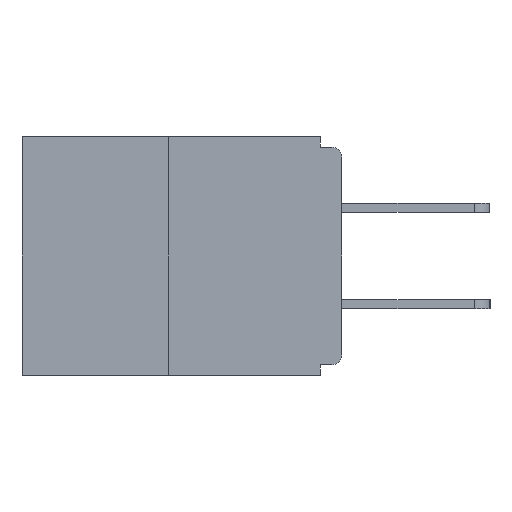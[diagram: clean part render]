
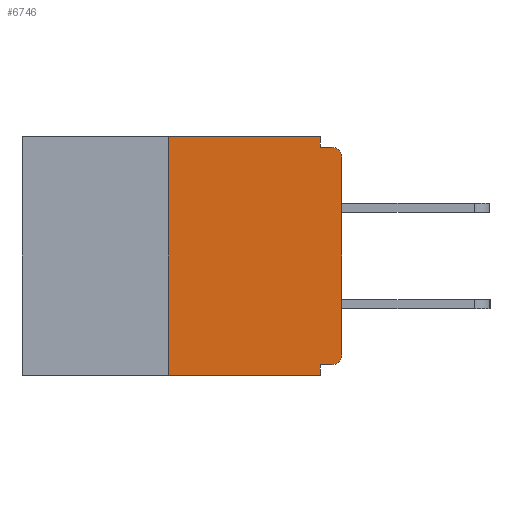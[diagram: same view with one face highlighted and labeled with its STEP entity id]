
A CAD part, left-side view. The second image highlights one B-rep face of the part: STEP entity #6746.
In plain terms, the highlighted planar face has unit normal (-1, 0, 0).
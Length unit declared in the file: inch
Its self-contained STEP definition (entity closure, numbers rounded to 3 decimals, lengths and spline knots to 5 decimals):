
#115 = EDGE_LOOP ( 'NONE', ( #3226, #12368, #12212, #9473, #7868, #4380, #4260, #8943, #7143, #5866 ) ) ;
#445 = DIRECTION ( 'NONE',  ( 0., -1., 0. ) ) ;
#654 = VECTOR ( 'NONE', #9874, 39.37008 ) ;
#875 = CARTESIAN_POINT ( 'NONE',  ( 0., 0., 0. ) ) ;
#1223 = EDGE_CURVE ( 'NONE', #3018, #7444, #6487, .T. ) ;
#1386 = VERTEX_POINT ( 'NONE', #5911 ) ;
#1626 = CARTESIAN_POINT ( 'NONE',  ( 0., 0., -0.03 ) ) ;
#1693 = CIRCLE ( 'NONE', #7611, 0.015 ) ;
#1786 = VECTOR ( 'NONE', #445, 39.37008 ) ;
#2025 = VERTEX_POINT ( 'NONE', #10905 ) ;
#2146 = CARTESIAN_POINT ( 'NONE',  ( 0., 0.015, -0.015 ) ) ;
#2231 = EDGE_CURVE ( 'NONE', #6453, #13157, #6046, .T. ) ;
#2232 = EDGE_CURVE ( 'NONE', #4487, #3018, #13692, .T. ) ;
#2355 = CARTESIAN_POINT ( 'NONE',  ( 0., 0.015, -0.03 ) ) ;
#2812 = DIRECTION ( 'NONE',  ( 0., 0., -1. ) ) ;
#2990 = LINE ( 'NONE', #7348, #11748 ) ;
#2993 = EDGE_CURVE ( 'NONE', #1386, #13157, #13668, .T. ) ;
#3010 = LINE ( 'NONE', #7367, #12233 ) ;
#3018 = VERTEX_POINT ( 'NONE', #1626 ) ;
#3226 = ORIENTED_EDGE ( 'NONE', *, *, #5640, .F. ) ;
#3436 = EDGE_CURVE ( 'NONE', #2025, #4487, #1693, .T. ) ;
#3664 = PLANE ( 'NONE',  #12753 ) ;
#3708 = EDGE_CURVE ( 'NONE', #8237, #4792, #5709, .T. ) ;
#3715 = VECTOR ( 'NONE', #2812, 39.37008 ) ;
#3766 = LINE ( 'NONE', #12398, #1786 ) ;
#3793 = DIRECTION ( 'NONE',  ( 1., 0., 0. ) ) ;
#4013 = EDGE_CURVE ( 'NONE', #4792, #7444, #9715, .T. ) ;
#4260 = ORIENTED_EDGE ( 'NONE', *, *, #2232, .T. ) ;
#4293 = DIRECTION ( 'NONE',  ( 0., 0., -1. ) ) ;
#4380 = ORIENTED_EDGE ( 'NONE', *, *, #3436, .T. ) ;
#4487 = VERTEX_POINT ( 'NONE', #13026 ) ;
#4792 = VERTEX_POINT ( 'NONE', #13716 ) ;
#4859 = CARTESIAN_POINT ( 'NONE',  ( 0., 0.46, 0. ) ) ;
#4881 = AXIS2_PLACEMENT_3D ( 'NONE', #2355, #11877, #13211 ) ;
#4924 = EDGE_CURVE ( 'NONE', #2025, #1386, #3010, .T. ) ;
#5147 = DIRECTION ( 'NONE',  ( -1., 0., 0. ) ) ;
#5640 = EDGE_CURVE ( 'NONE', #11037, #8237, #3766, .T. ) ;
#5709 = LINE ( 'NONE', #8798, #654 ) ;
#5866 = ORIENTED_EDGE ( 'NONE', *, *, #3708, .F. ) ;
#5911 = CARTESIAN_POINT ( 'NONE',  ( 0., 0.031, -0.328 ) ) ;
#6046 = LINE ( 'NONE', #7124, #10108 ) ;
#6074 = CARTESIAN_POINT ( 'NONE',  ( 0., 0.015, -0.313 ) ) ;
#6453 = VERTEX_POINT ( 'NONE', #7529 ) ;
#6487 = CIRCLE ( 'NONE', #4881, 0.015 ) ;
#6696 = CARTESIAN_POINT ( 'NONE',  ( 0., 0.25, 0. ) ) ;
#6746 = ADVANCED_FACE ( 'NONE', ( #9229 ), #3664, .F. ) ;
#7124 = CARTESIAN_POINT ( 'NONE',  ( 0., 0.46, -0.343 ) ) ;
#7143 = ORIENTED_EDGE ( 'NONE', *, *, #4013, .F. ) ;
#7348 = CARTESIAN_POINT ( 'NONE',  ( 0., 0.25, 0. ) ) ;
#7367 = CARTESIAN_POINT ( 'NONE',  ( 0., 0., -0.328 ) ) ;
#7444 = VERTEX_POINT ( 'NONE', #2146 ) ;
#7529 = CARTESIAN_POINT ( 'NONE',  ( 0., 0.25, -0.343 ) ) ;
#7544 = CARTESIAN_POINT ( 'NONE',  ( 0., 0.031, -0.343 ) ) ;
#7611 = AXIS2_PLACEMENT_3D ( 'NONE', #6074, #5147, #4293 ) ;
#7868 = ORIENTED_EDGE ( 'NONE', *, *, #4924, .F. ) ;
#8237 = VERTEX_POINT ( 'NONE', #9869 ) ;
#8421 = DIRECTION ( 'NONE',  ( 0., -1., 0. ) ) ;
#8643 = CARTESIAN_POINT ( 'NONE',  ( 0., 0., -0.015 ) ) ;
#8655 = DIRECTION ( 'NONE',  ( 0., 1., 0. ) ) ;
#8798 = CARTESIAN_POINT ( 'NONE',  ( 0., 0.031, 0. ) ) ;
#8943 = ORIENTED_EDGE ( 'NONE', *, *, #1223, .T. ) ;
#9164 = DIRECTION ( 'NONE',  ( 0., 0., -1. ) ) ;
#9229 = FACE_OUTER_BOUND ( 'NONE', #115, .T. ) ;
#9473 = ORIENTED_EDGE ( 'NONE', *, *, #2993, .F. ) ;
#9715 = LINE ( 'NONE', #8643, #11116 ) ;
#9869 = CARTESIAN_POINT ( 'NONE',  ( 0., 0.031, 0. ) ) ;
#9874 = DIRECTION ( 'NONE',  ( 0., 0., -1. ) ) ;
#10108 = VECTOR ( 'NONE', #8421, 39.37008 ) ;
#10905 = CARTESIAN_POINT ( 'NONE',  ( 0., 0.015, -0.328 ) ) ;
#10976 = EDGE_CURVE ( 'NONE', #6453, #11037, #2990, .T. ) ;
#11037 = VERTEX_POINT ( 'NONE', #6696 ) ;
#11116 = VECTOR ( 'NONE', #14056, 39.37008 ) ;
#11706 = DIRECTION ( 'NONE',  ( 0., 0., 1. ) ) ;
#11748 = VECTOR ( 'NONE', #11706, 39.37008 ) ;
#11877 = DIRECTION ( 'NONE',  ( -1., 0., 0. ) ) ;
#12212 = ORIENTED_EDGE ( 'NONE', *, *, #2231, .T. ) ;
#12233 = VECTOR ( 'NONE', #8655, 39.37008 ) ;
#12368 = ORIENTED_EDGE ( 'NONE', *, *, #10976, .F. ) ;
#12398 = CARTESIAN_POINT ( 'NONE',  ( 0., 0.46, 0. ) ) ;
#12753 = AXIS2_PLACEMENT_3D ( 'NONE', #4859, #3793, #9164 ) ;
#12764 = DIRECTION ( 'NONE',  ( 0., 0., 1. ) ) ;
#13026 = CARTESIAN_POINT ( 'NONE',  ( 0., 0., -0.313 ) ) ;
#13157 = VERTEX_POINT ( 'NONE', #7544 ) ;
#13211 = DIRECTION ( 'NONE',  ( 0., 0., -1. ) ) ;
#13668 = LINE ( 'NONE', #13738, #3715 ) ;
#13692 = LINE ( 'NONE', #875, #13736 ) ;
#13716 = CARTESIAN_POINT ( 'NONE',  ( 0., 0.031, -0.015 ) ) ;
#13736 = VECTOR ( 'NONE', #12764, 39.37008 ) ;
#13738 = CARTESIAN_POINT ( 'NONE',  ( 0., 0.031, -0.343 ) ) ;
#14056 = DIRECTION ( 'NONE',  ( 0., -1., 0. ) ) ;
